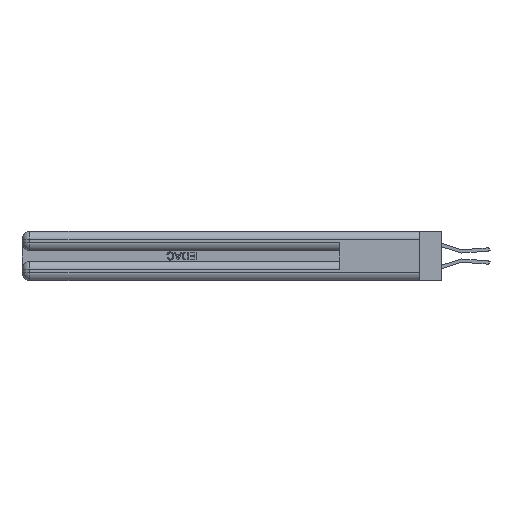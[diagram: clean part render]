
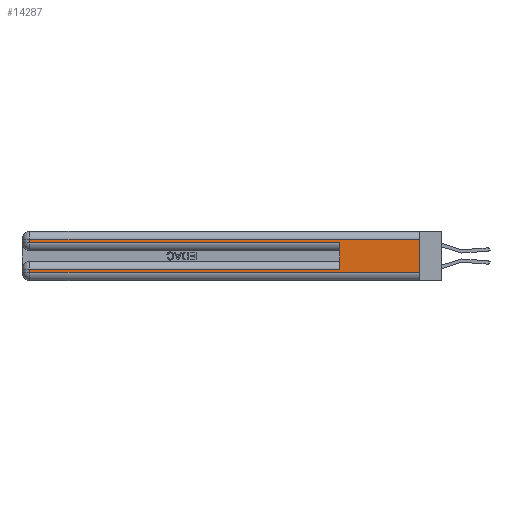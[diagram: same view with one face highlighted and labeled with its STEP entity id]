
A CAD part, left-side view. The second image highlights one B-rep face of the part: STEP entity #14287.
In plain terms, the highlighted planar face has unit normal (-1, 0, 0).
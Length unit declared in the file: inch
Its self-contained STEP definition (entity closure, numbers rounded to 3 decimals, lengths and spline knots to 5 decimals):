
#83 = EDGE_CURVE ( 'NONE', #22012, #41620, #27061, .T. ) ;
#381 = VECTOR ( 'NONE', #28489, 39.37008 ) ;
#2664 = VECTOR ( 'NONE', #34523, 39.37008 ) ;
#2925 = CARTESIAN_POINT ( 'NONE',  ( 0., 0., 0.06 ) ) ;
#3471 = EDGE_CURVE ( 'NONE', #15181, #29704, #36437, .T. ) ;
#5826 = CARTESIAN_POINT ( 'NONE',  ( 0., 0., 0.06 ) ) ;
#5867 = DIRECTION ( 'NONE',  ( 0., 0., -1. ) ) ;
#6002 = CARTESIAN_POINT ( 'NONE',  ( 0., 2.94, 0.085 ) ) ;
#6209 = DIRECTION ( 'NONE',  ( 0., 0., 1. ) ) ;
#6237 = ORIENTED_EDGE ( 'NONE', *, *, #3471, .F. ) ;
#6261 = DIRECTION ( 'NONE',  ( 0., -1., 0. ) ) ;
#6670 = ORIENTED_EDGE ( 'NONE', *, *, #38815, .F. ) ;
#7957 = CARTESIAN_POINT ( 'NONE',  ( 0., 2.94, 0.285 ) ) ;
#9887 = ORIENTED_EDGE ( 'NONE', *, *, #83, .T. ) ;
#10463 = VECTOR ( 'NONE', #5867, 39.37008 ) ;
#11084 = VERTEX_POINT ( 'NONE', #6002 ) ;
#12059 = CARTESIAN_POINT ( 'NONE',  ( 0., 2.94, 0.31 ) ) ;
#13648 = ORIENTED_EDGE ( 'NONE', *, *, #40048, .T. ) ;
#13833 = CARTESIAN_POINT ( 'NONE',  ( 0., 2.94, 0.37 ) ) ;
#13890 = LINE ( 'NONE', #31259, #2664 ) ;
#14005 = DIRECTION ( 'NONE',  ( 1., 0., 0. ) ) ;
#14287 = ADVANCED_FACE ( 'NONE', ( #38467 ), #17358, .F. ) ;
#15181 = VERTEX_POINT ( 'NONE', #17117 ) ;
#15653 = VECTOR ( 'NONE', #41225, 39.37008 ) ;
#15663 = CARTESIAN_POINT ( 'NONE',  ( 0., 2.94, 0.37 ) ) ;
#16395 = ORIENTED_EDGE ( 'NONE', *, *, #21249, .T. ) ;
#16635 = DIRECTION ( 'NONE',  ( 0., 0., -1. ) ) ;
#16716 = LINE ( 'NONE', #15663, #381 ) ;
#17117 = CARTESIAN_POINT ( 'NONE',  ( 0., 0., 0.31 ) ) ;
#17358 = PLANE ( 'NONE',  #25121 ) ;
#18654 = CARTESIAN_POINT ( 'NONE',  ( 0., 0.6, 0.085 ) ) ;
#20590 = LINE ( 'NONE', #5826, #36862 ) ;
#21222 = VERTEX_POINT ( 'NONE', #18654 ) ;
#21249 = EDGE_CURVE ( 'NONE', #11084, #36967, #16716, .T. ) ;
#22012 = VERTEX_POINT ( 'NONE', #7957 ) ;
#22299 = CARTESIAN_POINT ( 'NONE',  ( 0., 2.94, 0.06 ) ) ;
#23322 = EDGE_CURVE ( 'NONE', #21222, #11084, #37522, .T. ) ;
#23535 = CARTESIAN_POINT ( 'NONE',  ( 0., 0., 0.285 ) ) ;
#23995 = CARTESIAN_POINT ( 'NONE',  ( 0., 0.6, 0.285 ) ) ;
#25121 = AXIS2_PLACEMENT_3D ( 'NONE', #33467, #14005, #40185 ) ;
#26452 = LINE ( 'NONE', #13833, #27653 ) ;
#26519 = VERTEX_POINT ( 'NONE', #12059 ) ;
#27061 = LINE ( 'NONE', #23535, #40884 ) ;
#27653 = VECTOR ( 'NONE', #16635, 39.37008 ) ;
#27752 = VECTOR ( 'NONE', #6209, 39.37008 ) ;
#28489 = DIRECTION ( 'NONE',  ( 0., 0., -1. ) ) ;
#28816 = LINE ( 'NONE', #38952, #27752 ) ;
#29205 = EDGE_CURVE ( 'NONE', #26519, #22012, #26452, .T. ) ;
#29704 = VERTEX_POINT ( 'NONE', #2925 ) ;
#29712 = ORIENTED_EDGE ( 'NONE', *, *, #32860, .T. ) ;
#30893 = DIRECTION ( 'NONE',  ( 0., -1., 0. ) ) ;
#31259 = CARTESIAN_POINT ( 'NONE',  ( 0., 0., 0.31 ) ) ;
#32860 = EDGE_CURVE ( 'NONE', #36967, #29704, #20590, .T. ) ;
#32927 = ORIENTED_EDGE ( 'NONE', *, *, #29205, .T. ) ;
#33467 = CARTESIAN_POINT ( 'NONE',  ( 0., 0., 0.37 ) ) ;
#34523 = DIRECTION ( 'NONE',  ( 0., 1., 0. ) ) ;
#36437 = LINE ( 'NONE', #38343, #10463 ) ;
#36862 = VECTOR ( 'NONE', #6261, 39.37008 ) ;
#36967 = VERTEX_POINT ( 'NONE', #22299 ) ;
#37522 = LINE ( 'NONE', #37916, #15653 ) ;
#37916 = CARTESIAN_POINT ( 'NONE',  ( 0., 0., 0.085 ) ) ;
#38343 = CARTESIAN_POINT ( 'NONE',  ( 0., 0., 0.37 ) ) ;
#38467 = FACE_OUTER_BOUND ( 'NONE', #40600, .T. ) ;
#38815 = EDGE_CURVE ( 'NONE', #21222, #41620, #28816, .T. ) ;
#38952 = CARTESIAN_POINT ( 'NONE',  ( 0., 0.6, 0.145 ) ) ;
#40048 = EDGE_CURVE ( 'NONE', #15181, #26519, #13890, .T. ) ;
#40185 = DIRECTION ( 'NONE',  ( 0., 0., -1. ) ) ;
#40600 = EDGE_LOOP ( 'NONE', ( #6237, #13648, #32927, #9887, #6670, #41515, #16395, #29712 ) ) ;
#40884 = VECTOR ( 'NONE', #30893, 39.37008 ) ;
#41225 = DIRECTION ( 'NONE',  ( 0., 1., 0. ) ) ;
#41515 = ORIENTED_EDGE ( 'NONE', *, *, #23322, .T. ) ;
#41620 = VERTEX_POINT ( 'NONE', #23995 ) ;
